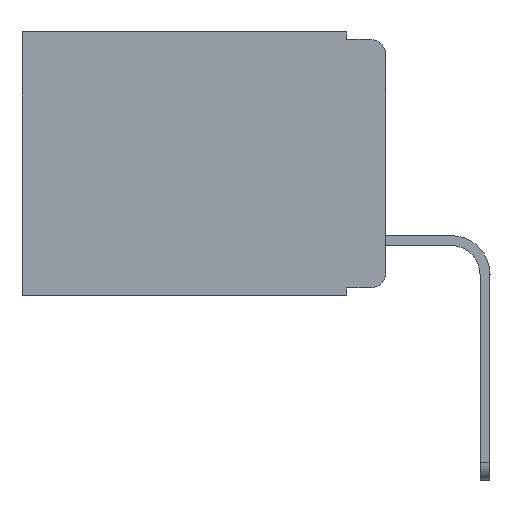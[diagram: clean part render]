
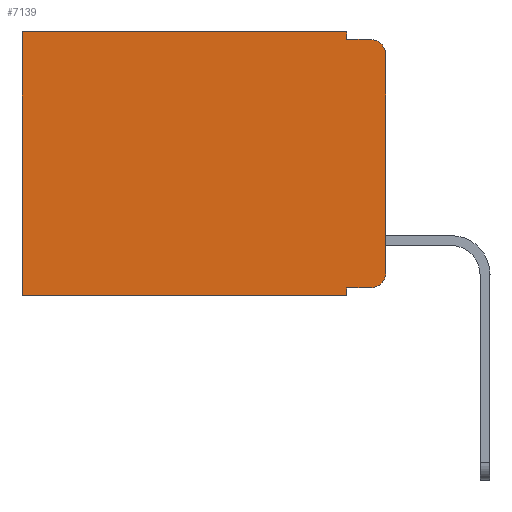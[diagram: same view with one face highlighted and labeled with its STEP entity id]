
A CAD part, left-side view. The second image highlights one B-rep face of the part: STEP entity #7139.
In plain terms, the highlighted planar face has unit normal (-1, 0, 0).
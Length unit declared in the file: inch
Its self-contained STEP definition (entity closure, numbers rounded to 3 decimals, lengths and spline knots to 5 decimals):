
#163 = CARTESIAN_POINT ( 'NONE',  ( 0.298, 0.02, -0.313 ) ) ;
#177 = DIRECTION ( 'NONE',  ( 1., 0., 0. ) ) ;
#244 = EDGE_CURVE ( 'NONE', #9665, #810, #492, .T. ) ;
#492 = LINE ( 'NONE', #5106, #1960 ) ;
#521 = EDGE_CURVE ( 'NONE', #9452, #813, #4952, .T. ) ;
#546 = EDGE_CURVE ( 'NONE', #9665, #1511, #6032, .T. ) ;
#629 = CARTESIAN_POINT ( 'NONE',  ( 0.298, 0., -0.343 ) ) ;
#767 = CIRCLE ( 'NONE', #8761, 0.02 ) ;
#810 = VERTEX_POINT ( 'NONE', #5412 ) ;
#813 = VERTEX_POINT ( 'NONE', #8616 ) ;
#944 = FACE_OUTER_BOUND ( 'NONE', #3997, .T. ) ;
#1252 = DIRECTION ( 'NONE',  ( -1., 0., 0. ) ) ;
#1511 = VERTEX_POINT ( 'NONE', #8417 ) ;
#1591 = LINE ( 'NONE', #1672, #4998 ) ;
#1651 = CARTESIAN_POINT ( 'NONE',  ( 0.298, 0., -0.03 ) ) ;
#1672 = CARTESIAN_POINT ( 'NONE',  ( 0.298, 0.051, 0. ) ) ;
#1821 = DIRECTION ( 'NONE',  ( 0., -1., 0. ) ) ;
#1955 = LINE ( 'NONE', #629, #3403 ) ;
#1960 = VECTOR ( 'NONE', #2754, 39.37008 ) ;
#2030 = DIRECTION ( 'NONE',  ( 0., 0., -1. ) ) ;
#2106 = VECTOR ( 'NONE', #7717, 39.37008 ) ;
#2443 = ORIENTED_EDGE ( 'NONE', *, *, #521, .F. ) ;
#2526 = DIRECTION ( 'NONE',  ( -1., 0., 0. ) ) ;
#2663 = CARTESIAN_POINT ( 'NONE',  ( 0.298, 0.051, -0.333 ) ) ;
#2754 = DIRECTION ( 'NONE',  ( 0., 0., -1. ) ) ;
#3224 = DIRECTION ( 'NONE',  ( 0., 0., -1. ) ) ;
#3403 = VECTOR ( 'NONE', #9224, 39.37008 ) ;
#3507 = ORIENTED_EDGE ( 'NONE', *, *, #5046, .F. ) ;
#3997 = EDGE_LOOP ( 'NONE', ( #2443, #9653, #9427, #5289, #9770, #6657, #4335, #3507, #9710, #5969 ) ) ;
#4169 = EDGE_CURVE ( 'NONE', #5684, #8717, #1955, .T. ) ;
#4333 = VECTOR ( 'NONE', #9829, 39.37008 ) ;
#4335 = ORIENTED_EDGE ( 'NONE', *, *, #4169, .F. ) ;
#4547 = EDGE_CURVE ( 'NONE', #7922, #4864, #9335, .T. ) ;
#4864 = VERTEX_POINT ( 'NONE', #6986 ) ;
#4952 = LINE ( 'NONE', #9073, #4333 ) ;
#4998 = VECTOR ( 'NONE', #8944, 39.37008 ) ;
#5046 = EDGE_CURVE ( 'NONE', #7922, #5684, #1591, .T. ) ;
#5106 = CARTESIAN_POINT ( 'NONE',  ( 0.298, 0.051, 0. ) ) ;
#5205 = VERTEX_POINT ( 'NONE', #5662 ) ;
#5289 = ORIENTED_EDGE ( 'NONE', *, *, #244, .F. ) ;
#5355 = VECTOR ( 'NONE', #1821, 39.37008 ) ;
#5412 = CARTESIAN_POINT ( 'NONE',  ( 0.298, 0.051, -0.01 ) ) ;
#5567 = PLANE ( 'NONE',  #6264 ) ;
#5662 = CARTESIAN_POINT ( 'NONE',  ( 0.298, 0.02, -0.01 ) ) ;
#5684 = VERTEX_POINT ( 'NONE', #9751 ) ;
#5694 = CARTESIAN_POINT ( 'NONE',  ( 0.298, 0.051, 0. ) ) ;
#5969 = ORIENTED_EDGE ( 'NONE', *, *, #9993, .T. ) ;
#6032 = LINE ( 'NONE', #8307, #10128 ) ;
#6044 = CARTESIAN_POINT ( 'NONE',  ( 0.298, 0.473, -0.343 ) ) ;
#6264 = AXIS2_PLACEMENT_3D ( 'NONE', #8842, #177, #3224 ) ;
#6641 = DIRECTION ( 'NONE',  ( 0., 1., 0. ) ) ;
#6657 = ORIENTED_EDGE ( 'NONE', *, *, #9832, .T. ) ;
#6712 = CARTESIAN_POINT ( 'NONE',  ( 0.298, 0.02, -0.03 ) ) ;
#6824 = AXIS2_PLACEMENT_3D ( 'NONE', #6712, #1252, #2030 ) ;
#6986 = CARTESIAN_POINT ( 'NONE',  ( 0.298, 0.02, -0.333 ) ) ;
#6990 = CARTESIAN_POINT ( 'NONE',  ( 0.298, 0.473, 0. ) ) ;
#7139 = ADVANCED_FACE ( 'NONE', ( #944 ), #5567, .F. ) ;
#7247 = CIRCLE ( 'NONE', #6824, 0.02 ) ;
#7717 = DIRECTION ( 'NONE',  ( 0., 0., -1. ) ) ;
#7869 = CARTESIAN_POINT ( 'NONE',  ( 0.298, 0.051, -0.01 ) ) ;
#7922 = VERTEX_POINT ( 'NONE', #8154 ) ;
#8154 = CARTESIAN_POINT ( 'NONE',  ( 0.298, 0.051, -0.333 ) ) ;
#8242 = LINE ( 'NONE', #6990, #2106 ) ;
#8307 = CARTESIAN_POINT ( 'NONE',  ( 0.298, 0., 0. ) ) ;
#8417 = CARTESIAN_POINT ( 'NONE',  ( 0.298, 0.473, 0. ) ) ;
#8502 = LINE ( 'NONE', #7869, #9113 ) ;
#8587 = DIRECTION ( 'NONE',  ( 0., -1., 0. ) ) ;
#8616 = CARTESIAN_POINT ( 'NONE',  ( 0.298, 0., -0.313 ) ) ;
#8717 = VERTEX_POINT ( 'NONE', #6044 ) ;
#8761 = AXIS2_PLACEMENT_3D ( 'NONE', #163, #2526, #9472 ) ;
#8842 = CARTESIAN_POINT ( 'NONE',  ( 0.298, 0., 0. ) ) ;
#8944 = DIRECTION ( 'NONE',  ( 0., 0., -1. ) ) ;
#9073 = CARTESIAN_POINT ( 'NONE',  ( 0.298, 0., 0. ) ) ;
#9102 = EDGE_CURVE ( 'NONE', #9452, #5205, #7247, .T. ) ;
#9113 = VECTOR ( 'NONE', #8587, 39.37008 ) ;
#9224 = DIRECTION ( 'NONE',  ( 0., 1., 0. ) ) ;
#9335 = LINE ( 'NONE', #2663, #5355 ) ;
#9357 = EDGE_CURVE ( 'NONE', #810, #5205, #8502, .T. ) ;
#9427 = ORIENTED_EDGE ( 'NONE', *, *, #9357, .F. ) ;
#9452 = VERTEX_POINT ( 'NONE', #1651 ) ;
#9472 = DIRECTION ( 'NONE',  ( 0., 0., -1. ) ) ;
#9653 = ORIENTED_EDGE ( 'NONE', *, *, #9102, .T. ) ;
#9665 = VERTEX_POINT ( 'NONE', #5694 ) ;
#9710 = ORIENTED_EDGE ( 'NONE', *, *, #4547, .T. ) ;
#9751 = CARTESIAN_POINT ( 'NONE',  ( 0.298, 0.051, -0.343 ) ) ;
#9770 = ORIENTED_EDGE ( 'NONE', *, *, #546, .T. ) ;
#9829 = DIRECTION ( 'NONE',  ( 0., 0., -1. ) ) ;
#9832 = EDGE_CURVE ( 'NONE', #1511, #8717, #8242, .T. ) ;
#9993 = EDGE_CURVE ( 'NONE', #4864, #813, #767, .T. ) ;
#10128 = VECTOR ( 'NONE', #6641, 39.37008 ) ;
